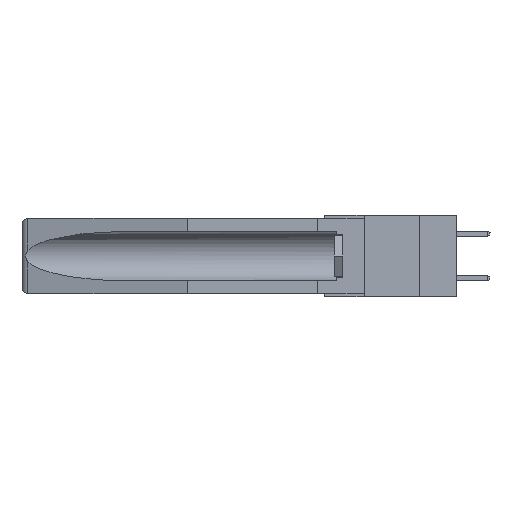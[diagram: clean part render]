
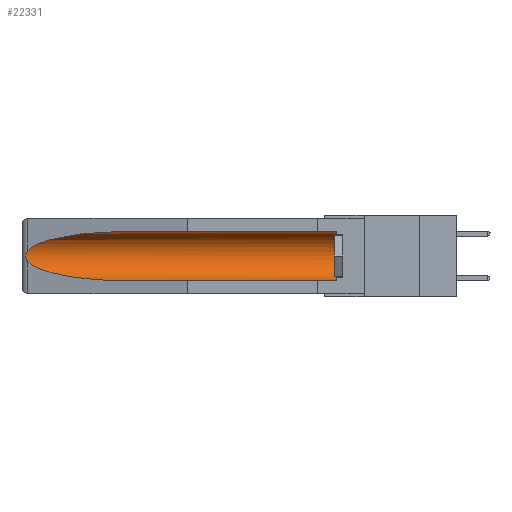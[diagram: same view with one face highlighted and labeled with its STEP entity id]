
A CAD part, left-side view. The second image highlights one B-rep face of the part: STEP entity #22331.
In plain terms, the highlighted cylindrical face has radius 2.857 mm (diameter 5.715 mm), a partial arc.
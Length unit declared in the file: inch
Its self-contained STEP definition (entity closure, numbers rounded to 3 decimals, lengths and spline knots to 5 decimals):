
#155 = DIRECTION ( 'NONE',  ( 0., -1., 0. ) ) ;
#593 = AXIS2_PLACEMENT_3D ( 'NONE', #30923, #155, #17958 ) ;
#793 = B_SPLINE_CURVE_WITH_KNOTS ( 'NONE', 3,
 ( #1850, #27259, #9294, #11855, #14483, #4222, #6924, #19415, #24666, #16945 ),
 .UNSPECIFIED., .F., .F.,
 ( 4, 2, 2, 2, 4 ),
 ( 0., 0.00029, 0.00058, 0.00087, 0.00117 ),
 .UNSPECIFIED. ) ;
#1084 = EDGE_CURVE ( 'NONE', #32692, #1539, #20372, .T. ) ;
#1539 = VERTEX_POINT ( 'NONE', #27027 ) ;
#1850 = CARTESIAN_POINT ( 'NONE',  ( 0.26537, 1.52718, -0.14972 ) ) ;
#1910 = CARTESIAN_POINT ( 'NONE',  ( 0.155, 1.07973, -0.284 ) ) ;
#1969 = CARTESIAN_POINT ( 'NONE',  ( 0.25451, 1.48313, -0.09465 ) ) ;
#4222 = CARTESIAN_POINT ( 'NONE',  ( 0.2675, 1.53308, -0.17534 ) ) ;
#4511 = DIRECTION ( 'NONE',  ( 0., 1., 0. ) ) ;
#5396 = DIRECTION ( 'NONE',  ( 0., 1., 0. ) ) ;
#6335 = CARTESIAN_POINT ( 'NONE',  ( 0.21114, 1.30732, -0.284 ) ) ;
#6496 = EDGE_CURVE ( 'NONE', #19131, #10343, #26351, .T. ) ;
#6687 = CARTESIAN_POINT ( 'NONE',  ( 0.155, 0.126, -0.059 ) ) ;
#6924 = CARTESIAN_POINT ( 'NONE',  ( 0.2673, 1.53269, -0.17917 ) ) ;
#7985 = AXIS2_PLACEMENT_3D ( 'NONE', #18222, #5396, #23350 ) ;
#8303 = ORIENTED_EDGE ( 'NONE', *, *, #14242, .T. ) ;
#8570 = CARTESIAN_POINT ( 'NONE',  ( 0.155, 1.07973, -0.284 ) ) ;
#9007 = CARTESIAN_POINT ( 'NONE',  ( 0.155, 0.126, -0.284 ) ) ;
#9245 = EDGE_CURVE ( 'NONE', #1539, #15580, #793, .T. ) ;
#9294 = CARTESIAN_POINT ( 'NONE',  ( 0.26654, 1.53092, -0.15636 ) ) ;
#10343 = VERTEX_POINT ( 'NONE', #6687 ) ;
#11345 = EDGE_CURVE ( 'NONE', #10343, #32692, #11377, .T. ) ;
#11377 = LINE ( 'NONE', #31725, #19426 ) ;
#11855 = CARTESIAN_POINT ( 'NONE',  ( 0.2673, 1.5327, -0.16383 ) ) ;
#12094 = VECTOR ( 'NONE', #4511, 39.37008 ) ;
#12096 = CARTESIAN_POINT ( 'NONE',  ( 0.26537, 1.52718, -0.14972 ) ) ;
#12218 = CARTESIAN_POINT ( 'NONE',  ( 0.155, 1.07973, -0.059 ) ) ;
#12265 = CARTESIAN_POINT ( 'NONE',  ( 0.155, -0.30754, -0.284 ) ) ;
#13203 =( BOUNDED_CURVE ( )  B_SPLINE_CURVE ( 3, ( #26870, #32009, #6335, #8570 ),
 .UNSPECIFIED., .F., .F. ) 
 B_SPLINE_CURVE_WITH_KNOTS ( ( 4, 4 ),
 ( 0.1948, 1.5708 ),
 .UNSPECIFIED. ) 
 CURVE ( )  GEOMETRIC_REPRESENTATION_ITEM ( )  RATIONAL_B_SPLINE_CURVE ( ( 1., 0.848, 0.848, 1. ) ) 
 REPRESENTATION_ITEM ( '' )  );
#14242 = EDGE_CURVE ( 'NONE', #15580, #32317, #13203, .T. ) ;
#14483 = CARTESIAN_POINT ( 'NONE',  ( 0.2675, 1.53308, -0.16763 ) ) ;
#15580 = VERTEX_POINT ( 'NONE', #29737 ) ;
#16912 = CYLINDRICAL_SURFACE ( 'NONE', #7985, 0.1125 ) ;
#16945 = CARTESIAN_POINT ( 'NONE',  ( 0.26537, 1.52718, -0.19328 ) ) ;
#17958 = DIRECTION ( 'NONE',  ( 0., 0., 1. ) ) ;
#18222 = CARTESIAN_POINT ( 'NONE',  ( 0.155, -0.30754, -0.1715 ) ) ;
#18525 = ORIENTED_EDGE ( 'NONE', *, *, #6496, .T. ) ;
#18743 = DIRECTION ( 'NONE',  ( 0., 1., 0. ) ) ;
#19131 = VERTEX_POINT ( 'NONE', #9007 ) ;
#19415 = CARTESIAN_POINT ( 'NONE',  ( 0.26655, 1.53094, -0.18657 ) ) ;
#19426 = VECTOR ( 'NONE', #18743, 39.37008 ) ;
#19841 = CARTESIAN_POINT ( 'NONE',  ( 0.155, 1.07973, -0.059 ) ) ;
#20372 =( BOUNDED_CURVE ( )  B_SPLINE_CURVE ( 3, ( #19841, #30243, #1969, #12096 ),
 .UNSPECIFIED., .F., .F. ) 
 B_SPLINE_CURVE_WITH_KNOTS ( ( 4, 4 ),
 ( 4.71239, 6.08839 ),
 .UNSPECIFIED. ) 
 CURVE ( )  GEOMETRIC_REPRESENTATION_ITEM ( )  RATIONAL_B_SPLINE_CURVE ( ( 1., 0.848, 0.848, 1. ) ) 
 REPRESENTATION_ITEM ( '' )  );
#20752 = ORIENTED_EDGE ( 'NONE', *, *, #1084, .T. ) ;
#22331 = ADVANCED_FACE ( 'NONE', ( #28913 ), #16912, .F. ) ;
#23350 = DIRECTION ( 'NONE',  ( 0., 0., 1. ) ) ;
#24666 = CARTESIAN_POINT ( 'NONE',  ( 0.26597, 1.5296, -0.19026 ) ) ;
#24706 = ORIENTED_EDGE ( 'NONE', *, *, #11345, .T. ) ;
#26351 = CIRCLE ( 'NONE', #593, 0.1125 ) ;
#26870 = CARTESIAN_POINT ( 'NONE',  ( 0.26537, 1.52718, -0.19328 ) ) ;
#27027 = CARTESIAN_POINT ( 'NONE',  ( 0.26537, 1.52718, -0.14972 ) ) ;
#27259 = CARTESIAN_POINT ( 'NONE',  ( 0.26597, 1.52961, -0.15275 ) ) ;
#27477 = EDGE_CURVE ( 'NONE', #19131, #32317, #27735, .T. ) ;
#27735 = LINE ( 'NONE', #12265, #12094 ) ;
#28565 = ORIENTED_EDGE ( 'NONE', *, *, #27477, .F. ) ;
#28913 = FACE_OUTER_BOUND ( 'NONE', #30826, .T. ) ;
#29737 = CARTESIAN_POINT ( 'NONE',  ( 0.26537, 1.52718, -0.19328 ) ) ;
#30243 = CARTESIAN_POINT ( 'NONE',  ( 0.21114, 1.30732, -0.059 ) ) ;
#30826 = EDGE_LOOP ( 'NONE', ( #20752, #32564, #8303, #28565, #18525, #24706 ) ) ;
#30923 = CARTESIAN_POINT ( 'NONE',  ( 0.155, 0.126, -0.1715 ) ) ;
#31725 = CARTESIAN_POINT ( 'NONE',  ( 0.155, -0.30754, -0.059 ) ) ;
#32009 = CARTESIAN_POINT ( 'NONE',  ( 0.25451, 1.48313, -0.24835 ) ) ;
#32317 = VERTEX_POINT ( 'NONE', #1910 ) ;
#32564 = ORIENTED_EDGE ( 'NONE', *, *, #9245, .T. ) ;
#32692 = VERTEX_POINT ( 'NONE', #12218 ) ;
